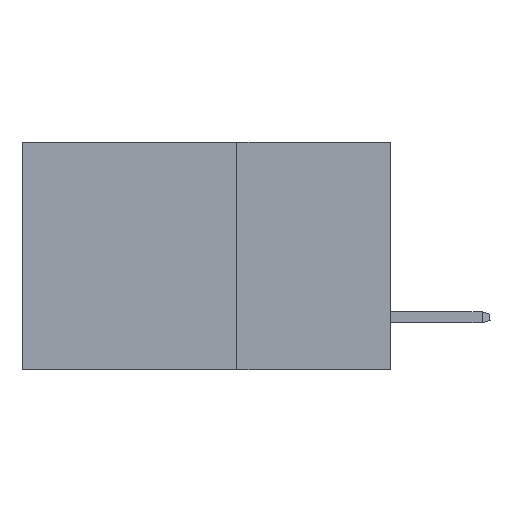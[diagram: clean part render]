
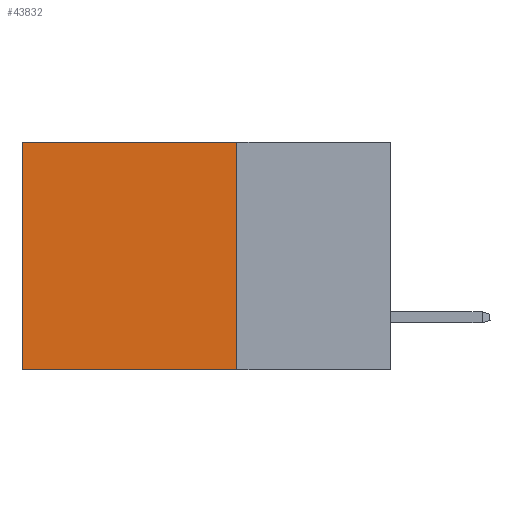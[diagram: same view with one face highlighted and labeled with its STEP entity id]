
A CAD part, left-side view. The second image highlights one B-rep face of the part: STEP entity #43832.
In plain terms, the highlighted planar face has unit normal (-1, 0, 0).
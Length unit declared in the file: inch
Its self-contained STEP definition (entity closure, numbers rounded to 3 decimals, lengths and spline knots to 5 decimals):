
#1628 = EDGE_LOOP ( 'NONE', ( #24966, #40522, #37302, #28762 ) ) ;
#3404 = FACE_OUTER_BOUND ( 'NONE', #1628, .T. ) ;
#4576 = CARTESIAN_POINT ( 'NONE',  ( 0.2875, 0.6, -0.37 ) ) ;
#5643 = VECTOR ( 'NONE', #30330, 39.37008 ) ;
#6775 = VECTOR ( 'NONE', #26901, 39.37008 ) ;
#7196 = VERTEX_POINT ( 'NONE', #8542 ) ;
#8174 = LINE ( 'NONE', #24196, #10303 ) ;
#8542 = CARTESIAN_POINT ( 'NONE',  ( 0.2875, 0.25, -0.37 ) ) ;
#9007 = PLANE ( 'NONE',  #22916 ) ;
#10035 = VERTEX_POINT ( 'NONE', #24605 ) ;
#10303 = VECTOR ( 'NONE', #20447, 39.37008 ) ;
#11035 = CARTESIAN_POINT ( 'NONE',  ( 0.2875, 0.25, 0. ) ) ;
#15559 = EDGE_CURVE ( 'NONE', #7196, #25987, #16783, .T. ) ;
#16260 = DIRECTION ( 'NONE',  ( 1., 0., 0. ) ) ;
#16783 = LINE ( 'NONE', #33452, #5643 ) ;
#18917 = VECTOR ( 'NONE', #29664, 39.37008 ) ;
#20447 = DIRECTION ( 'NONE',  ( 0., 1., 0. ) ) ;
#22386 = CARTESIAN_POINT ( 'NONE',  ( 0.2875, 0.6, 0. ) ) ;
#22916 = AXIS2_PLACEMENT_3D ( 'NONE', #26251, #16260, #40056 ) ;
#23451 = CARTESIAN_POINT ( 'NONE',  ( 0.2875, 0.25, 0. ) ) ;
#24196 = CARTESIAN_POINT ( 'NONE',  ( 0.2875, 0.25, 0. ) ) ;
#24605 = CARTESIAN_POINT ( 'NONE',  ( 0.2875, 0.6, 0. ) ) ;
#24966 = ORIENTED_EDGE ( 'NONE', *, *, #34701, .T. ) ;
#25762 = EDGE_CURVE ( 'NONE', #29744, #7196, #39242, .T. ) ;
#25987 = VERTEX_POINT ( 'NONE', #4576 ) ;
#26251 = CARTESIAN_POINT ( 'NONE',  ( 0.2875, 0.25, 0. ) ) ;
#26901 = DIRECTION ( 'NONE',  ( 0., 0., -1. ) ) ;
#28449 = EDGE_CURVE ( 'NONE', #29744, #10035, #8174, .T. ) ;
#28762 = ORIENTED_EDGE ( 'NONE', *, *, #28449, .T. ) ;
#29664 = DIRECTION ( 'NONE',  ( 0., 0., -1. ) ) ;
#29744 = VERTEX_POINT ( 'NONE', #11035 ) ;
#30330 = DIRECTION ( 'NONE',  ( 0., 1., 0. ) ) ;
#33452 = CARTESIAN_POINT ( 'NONE',  ( 0.2875, 0.25, -0.37 ) ) ;
#34701 = EDGE_CURVE ( 'NONE', #10035, #25987, #40247, .T. ) ;
#37302 = ORIENTED_EDGE ( 'NONE', *, *, #25762, .F. ) ;
#39242 = LINE ( 'NONE', #23451, #6775 ) ;
#40056 = DIRECTION ( 'NONE',  ( 0., 0., -1. ) ) ;
#40247 = LINE ( 'NONE', #22386, #18917 ) ;
#40522 = ORIENTED_EDGE ( 'NONE', *, *, #15559, .F. ) ;
#43832 = ADVANCED_FACE ( 'NONE', ( #3404 ), #9007, .F. ) ;
